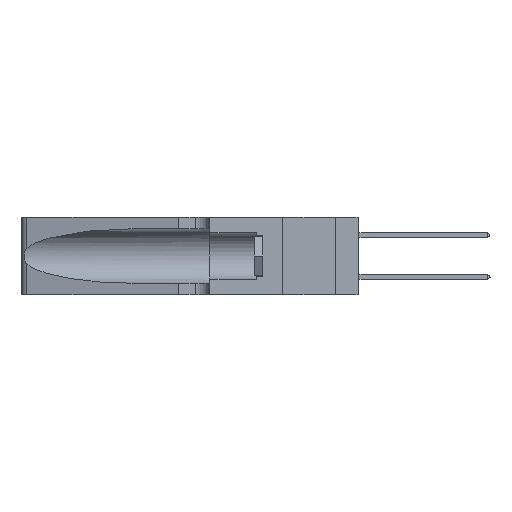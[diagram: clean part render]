
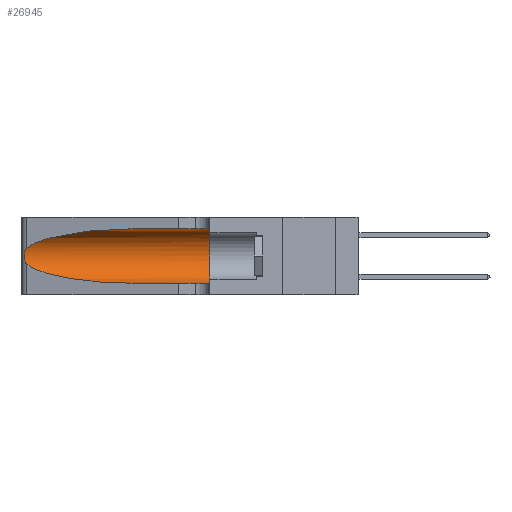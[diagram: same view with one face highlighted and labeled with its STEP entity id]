
A CAD part, left-side view. The second image highlights one B-rep face of the part: STEP entity #26945.
In plain terms, the highlighted cylindrical face has radius 3.308 mm (diameter 6.617 mm), a partial arc.
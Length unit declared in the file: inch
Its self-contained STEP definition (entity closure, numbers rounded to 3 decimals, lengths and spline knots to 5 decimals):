
#468 = DIRECTION ( 'NONE',  ( 0., 0., 1. ) ) ;
#757 = EDGE_CURVE ( 'NONE', #29690, #20401, #15191, .T. ) ;
#832 = CARTESIAN_POINT ( 'NONE',  ( 0.26075, 1.23896, 0.19203 ) ) ;
#845 = LINE ( 'NONE', #17029, #18843 ) ;
#1240 = EDGE_CURVE ( 'NONE', #9033, #15198, #14707, .T. ) ;
#2368 = CARTESIAN_POINT ( 'NONE',  ( 0.25487, 1.22718, 0.14631 ) ) ;
#3764 = CARTESIAN_POINT ( 'NONE',  ( 0.25487, 1.22718, 0.22369 ) ) ;
#3971 = DIRECTION ( 'NONE',  ( 0., -1., 0. ) ) ;
#4841 = AXIS2_PLACEMENT_3D ( 'NONE', #13771, #27136, #468 ) ;
#4988 = CARTESIAN_POINT ( 'NONE',  ( 0.25487, 1.22718, 0.14631 ) ) ;
#6244 = CARTESIAN_POINT ( 'NONE',  ( 0.1305, 1.61858, 0.31525 ) ) ;
#6434 = CARTESIAN_POINT ( 'NONE',  ( 0.25639, 1.23184, 0.21858 ) ) ;
#7365 = EDGE_CURVE ( 'NONE', #9466, #15198, #845, .T. ) ;
#7427 = ORIENTED_EDGE ( 'NONE', *, *, #7365, .T. ) ;
#7570 = VECTOR ( 'NONE', #19932, 39.37008 ) ;
#7600 = CARTESIAN_POINT ( 'NONE',  ( 0.25487, 1.22718, 0.22369 ) ) ;
#7671 = EDGE_LOOP ( 'NONE', ( #14347, #19879, #30025, #7427, #11815, #14947 ) ) ;
#8428 = LINE ( 'NONE', #6244, #7570 ) ;
#9033 = VERTEX_POINT ( 'NONE', #11944 ) ;
#9405 =( BOUNDED_CURVE ( )  B_SPLINE_CURVE ( 3, ( #25987, #17644, #12349, #23056 ),
 .UNSPECIFIED., .F., .F. ) 
 B_SPLINE_CURVE_WITH_KNOTS ( ( 4, 4 ),
 ( 1.5708, 2.84003 ),
 .UNSPECIFIED. ) 
 CURVE ( )  GEOMETRIC_REPRESENTATION_ITEM ( )  RATIONAL_B_SPLINE_CURVE ( ( 1., 0.87, 0.87, 1. ) ) 
 REPRESENTATION_ITEM ( '' )  );
#9466 = VERTEX_POINT ( 'NONE', #34482 ) ;
#10552 = EDGE_CURVE ( 'NONE', #24820, #29690, #9405, .T. ) ;
#10805 = CARTESIAN_POINT ( 'NONE',  ( 0.1305, 0.72297, 0.05475 ) ) ;
#11080 = DIRECTION ( 'NONE',  ( 0., -1., 0. ) ) ;
#11299 = AXIS2_PLACEMENT_3D ( 'NONE', #21773, #11080, #16569 ) ;
#11815 = ORIENTED_EDGE ( 'NONE', *, *, #1240, .F. ) ;
#11837 = CARTESIAN_POINT ( 'NONE',  ( 0.25856, 1.23593, 0.16098 ) ) ;
#11870 = CARTESIAN_POINT ( 'NONE',  ( 0.25555, 1.22994, 0.2215 ) ) ;
#11944 = CARTESIAN_POINT ( 'NONE',  ( 0.1305, 0.35, 0.31525 ) ) ;
#12349 = CARTESIAN_POINT ( 'NONE',  ( 0.2373, 1.15595, 0.28018 ) ) ;
#13771 = CARTESIAN_POINT ( 'NONE',  ( 0.1305, 0.35, 0.185 ) ) ;
#13793 = CARTESIAN_POINT ( 'NONE',  ( 0.25555, 1.22993, 0.14849 ) ) ;
#14347 = ORIENTED_EDGE ( 'NONE', *, *, #10552, .T. ) ;
#14707 = CIRCLE ( 'NONE', #4841, 0.13025 ) ;
#14947 = ORIENTED_EDGE ( 'NONE', *, *, #16604, .F. ) ;
#15191 = B_SPLINE_CURVE_WITH_KNOTS ( 'NONE', 3,
 ( #3764, #11870, #6434, #27602, #17291, #16830, #832, #27784, #20354, #11837, #20437, #19024, #13793, #2368 ),
 .UNSPECIFIED., .F., .F.,
 ( 4, 2, 2, 2, 2, 2, 4 ),
 ( 0., 0.00027, 0.00053, 0.00107, 0.0016, 0.00187, 0.00214 ),
 .UNSPECIFIED. ) ;
#15198 = VERTEX_POINT ( 'NONE', #21908 ) ;
#16569 = DIRECTION ( 'NONE',  ( 0., 0., -1. ) ) ;
#16600 = FACE_OUTER_BOUND ( 'NONE', #7671, .T. ) ;
#16604 = EDGE_CURVE ( 'NONE', #24820, #9033, #8428, .T. ) ;
#16830 = CARTESIAN_POINT ( 'NONE',  ( 0.26018, 1.23835, 0.19895 ) ) ;
#17029 = CARTESIAN_POINT ( 'NONE',  ( 0.1305, 1.61858, 0.05475 ) ) ;
#17291 = CARTESIAN_POINT ( 'NONE',  ( 0.25854, 1.2359, 0.20912 ) ) ;
#17644 = CARTESIAN_POINT ( 'NONE',  ( 0.18966, 0.96281, 0.31525 ) ) ;
#18843 = VECTOR ( 'NONE', #3971, 39.37008 ) ;
#19024 = CARTESIAN_POINT ( 'NONE',  ( 0.25639, 1.23186, 0.15144 ) ) ;
#19879 = ORIENTED_EDGE ( 'NONE', *, *, #757, .T. ) ;
#19932 = DIRECTION ( 'NONE',  ( 0., -1., 0. ) ) ;
#20354 = CARTESIAN_POINT ( 'NONE',  ( 0.26017, 1.23833, 0.17102 ) ) ;
#20401 = VERTEX_POINT ( 'NONE', #4988 ) ;
#20437 = CARTESIAN_POINT ( 'NONE',  ( 0.25789, 1.23486, 0.15765 ) ) ;
#20464 = EDGE_CURVE ( 'NONE', #20401, #9466, #26971, .T. ) ;
#21164 = CARTESIAN_POINT ( 'NONE',  ( 0.1305, 0.72297, 0.31525 ) ) ;
#21773 = CARTESIAN_POINT ( 'NONE',  ( 0.1305, 1.61858, 0.185 ) ) ;
#21908 = CARTESIAN_POINT ( 'NONE',  ( 0.1305, 0.35, 0.05475 ) ) ;
#23056 = CARTESIAN_POINT ( 'NONE',  ( 0.25487, 1.22718, 0.22369 ) ) ;
#24431 = CARTESIAN_POINT ( 'NONE',  ( 0.25487, 1.22718, 0.14631 ) ) ;
#24820 = VERTEX_POINT ( 'NONE', #21164 ) ;
#25987 = CARTESIAN_POINT ( 'NONE',  ( 0.1305, 0.72297, 0.31525 ) ) ;
#26869 = CARTESIAN_POINT ( 'NONE',  ( 0.18966, 0.96281, 0.05475 ) ) ;
#26945 = ADVANCED_FACE ( 'NONE', ( #16600 ), #29168, .F. ) ;
#26971 =( BOUNDED_CURVE ( )  B_SPLINE_CURVE ( 3, ( #24431, #29668, #26869, #10805 ),
 .UNSPECIFIED., .F., .T. ) 
 B_SPLINE_CURVE_WITH_KNOTS ( ( 4, 4 ),
 ( 3.44316, 4.71239 ),
 .UNSPECIFIED. ) 
 CURVE ( )  GEOMETRIC_REPRESENTATION_ITEM ( )  RATIONAL_B_SPLINE_CURVE ( ( 1., 0.87, 0.87, 1. ) ) 
 REPRESENTATION_ITEM ( '' )  );
#27136 = DIRECTION ( 'NONE',  ( 0., 1., 0. ) ) ;
#27602 = CARTESIAN_POINT ( 'NONE',  ( 0.25787, 1.23484, 0.2124 ) ) ;
#27784 = CARTESIAN_POINT ( 'NONE',  ( 0.26075, 1.23896, 0.178 ) ) ;
#29168 = CYLINDRICAL_SURFACE ( 'NONE', #11299, 0.13025 ) ;
#29668 = CARTESIAN_POINT ( 'NONE',  ( 0.2373, 1.15595, 0.08982 ) ) ;
#29690 = VERTEX_POINT ( 'NONE', #7600 ) ;
#30025 = ORIENTED_EDGE ( 'NONE', *, *, #20464, .T. ) ;
#34482 = CARTESIAN_POINT ( 'NONE',  ( 0.1305, 0.72297, 0.05475 ) ) ;
